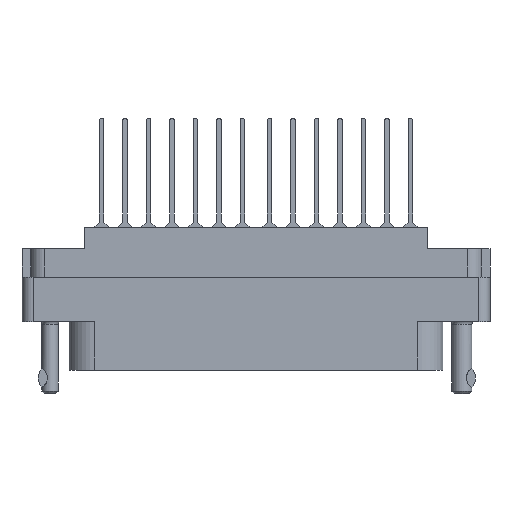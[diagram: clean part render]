
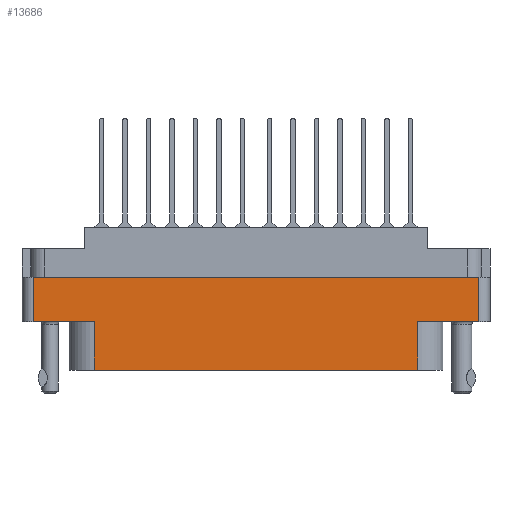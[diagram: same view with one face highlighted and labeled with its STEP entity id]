
A CAD part, front view. The second image highlights one B-rep face of the part: STEP entity #13686.
In plain terms, the highlighted planar face has unit normal (0, -1, 0).
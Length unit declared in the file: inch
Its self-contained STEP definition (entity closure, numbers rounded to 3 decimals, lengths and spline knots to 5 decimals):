
#203 = ORIENTED_EDGE ( 'NONE', *, *, #28921, .F. ) ;
#358 = LINE ( 'NONE', #29696, #55715 ) ;
#3760 = CARTESIAN_POINT ( 'NONE',  ( 0.895, -0.438, -0.52 ) ) ;
#6347 = EDGE_CURVE ( 'NONE', #36666, #17958, #37869, .T. ) ;
#6384 = ORIENTED_EDGE ( 'NONE', *, *, #34890, .T. ) ;
#6975 = DIRECTION ( 'NONE',  ( -1., 0., 0. ) ) ;
#12110 = CARTESIAN_POINT ( 'NONE',  ( 0.895, -0.438, -0.789 ) ) ;
#12327 = ORIENTED_EDGE ( 'NONE', *, *, #50824, .T. ) ;
#13070 = VERTEX_POINT ( 'NONE', #29493 ) ;
#13114 = EDGE_CURVE ( 'NONE', #46113, #13070, #21251, .T. ) ;
#13686 = ADVANCED_FACE ( 'NONE', ( #18356 ), #42509, .T. ) ;
#15303 = DIRECTION ( 'NONE',  ( 0., 0., 1. ) ) ;
#17958 = VERTEX_POINT ( 'NONE', #19154 ) ;
#18154 = VECTOR ( 'NONE', #48775, 39.37008 ) ;
#18356 = FACE_OUTER_BOUND ( 'NONE', #33194, .T. ) ;
#19154 = CARTESIAN_POINT ( 'NONE',  ( 0.895, -0.438, -0.52 ) ) ;
#19540 = LINE ( 'NONE', #35609, #33672 ) ;
#21251 = LINE ( 'NONE', #40118, #56715 ) ;
#21601 = DIRECTION ( 'NONE',  ( 0., 0., -1. ) ) ;
#21606 = DIRECTION ( 'NONE',  ( 0., -1., 0. ) ) ;
#21819 = CARTESIAN_POINT ( 'NONE',  ( -1.2335, -0.438, -0.274 ) ) ;
#23299 = DIRECTION ( 'NONE',  ( 1., 0., 0. ) ) ;
#23425 = VECTOR ( 'NONE', #6975, 39.37008 ) ;
#24702 = EDGE_CURVE ( 'NONE', #46113, #55497, #47582, .T. ) ;
#25057 = VECTOR ( 'NONE', #55399, 39.37008 ) ;
#25855 = ORIENTED_EDGE ( 'NONE', *, *, #37469, .T. ) ;
#26545 = LINE ( 'NONE', #51330, #41554 ) ;
#28821 = CARTESIAN_POINT ( 'NONE',  ( 0., -0.438, -0.274 ) ) ;
#28921 = EDGE_CURVE ( 'NONE', #50183, #40117, #51290, .T. ) ;
#29493 = CARTESIAN_POINT ( 'NONE',  ( -0.895, -0.438, -0.789 ) ) ;
#29696 = CARTESIAN_POINT ( 'NONE',  ( 1.2335, -0.438, -0.789 ) ) ;
#32820 = DIRECTION ( 'NONE',  ( 1., 0., 0. ) ) ;
#33194 = EDGE_LOOP ( 'NONE', ( #203, #25855, #38494, #58418, #6384, #37018, #55395, #12327 ) ) ;
#33672 = VECTOR ( 'NONE', #23299, 39.37008 ) ;
#34372 = CARTESIAN_POINT ( 'NONE',  ( 1.2335, -0.438, -0.52 ) ) ;
#34890 = EDGE_CURVE ( 'NONE', #13070, #51669, #19540, .T. ) ;
#35609 = CARTESIAN_POINT ( 'NONE',  ( -1.2955, -0.438, -0.789 ) ) ;
#35655 = VECTOR ( 'NONE', #32820, 39.37008 ) ;
#36666 = VERTEX_POINT ( 'NONE', #34372 ) ;
#37018 = ORIENTED_EDGE ( 'NONE', *, *, #39445, .T. ) ;
#37469 = EDGE_CURVE ( 'NONE', #50183, #55497, #26545, .T. ) ;
#37869 = LINE ( 'NONE', #46508, #25057 ) ;
#38494 = ORIENTED_EDGE ( 'NONE', *, *, #24702, .F. ) ;
#39445 = EDGE_CURVE ( 'NONE', #51669, #17958, #55718, .T. ) ;
#39504 = CARTESIAN_POINT ( 'NONE',  ( 1.2335, -0.438, -0.274 ) ) ;
#40117 = VERTEX_POINT ( 'NONE', #39504 ) ;
#40118 = CARTESIAN_POINT ( 'NONE',  ( -0.895, -0.438, -0.789 ) ) ;
#41554 = VECTOR ( 'NONE', #56077, 39.37008 ) ;
#41777 = CARTESIAN_POINT ( 'NONE',  ( -1.2335, -0.438, -0.52 ) ) ;
#42509 = PLANE ( 'NONE',  #46174 ) ;
#46113 = VERTEX_POINT ( 'NONE', #53114 ) ;
#46174 = AXIS2_PLACEMENT_3D ( 'NONE', #47078, #21606, #48818 ) ;
#46508 = CARTESIAN_POINT ( 'NONE',  ( 0., -0.438, -0.52 ) ) ;
#47078 = CARTESIAN_POINT ( 'NONE',  ( -1.2955, -0.438, -0.789 ) ) ;
#47582 = LINE ( 'NONE', #56526, #23425 ) ;
#48775 = DIRECTION ( 'NONE',  ( 0., 0., 1. ) ) ;
#48818 = DIRECTION ( 'NONE',  ( 0., 0., -1. ) ) ;
#50183 = VERTEX_POINT ( 'NONE', #21819 ) ;
#50824 = EDGE_CURVE ( 'NONE', #36666, #40117, #358, .T. ) ;
#51290 = LINE ( 'NONE', #28821, #35655 ) ;
#51330 = CARTESIAN_POINT ( 'NONE',  ( -1.2335, -0.438, -0.789 ) ) ;
#51669 = VERTEX_POINT ( 'NONE', #12110 ) ;
#53114 = CARTESIAN_POINT ( 'NONE',  ( -0.895, -0.438, -0.52 ) ) ;
#55395 = ORIENTED_EDGE ( 'NONE', *, *, #6347, .F. ) ;
#55399 = DIRECTION ( 'NONE',  ( -1., 0., 0. ) ) ;
#55497 = VERTEX_POINT ( 'NONE', #41777 ) ;
#55715 = VECTOR ( 'NONE', #15303, 39.37008 ) ;
#55718 = LINE ( 'NONE', #3760, #18154 ) ;
#56077 = DIRECTION ( 'NONE',  ( 0., 0., -1. ) ) ;
#56526 = CARTESIAN_POINT ( 'NONE',  ( 0., -0.438, -0.52 ) ) ;
#56715 = VECTOR ( 'NONE', #21601, 39.37008 ) ;
#58418 = ORIENTED_EDGE ( 'NONE', *, *, #13114, .T. ) ;
